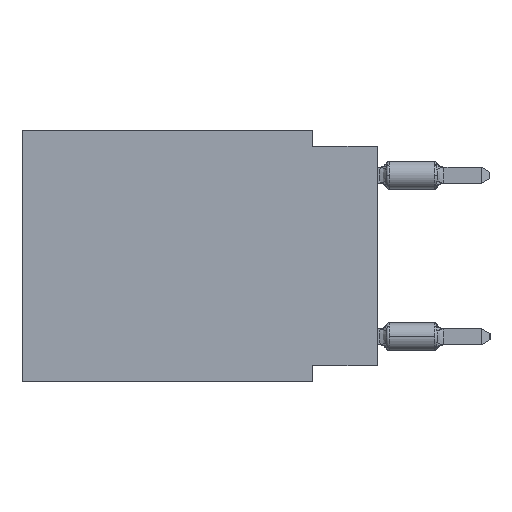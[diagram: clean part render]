
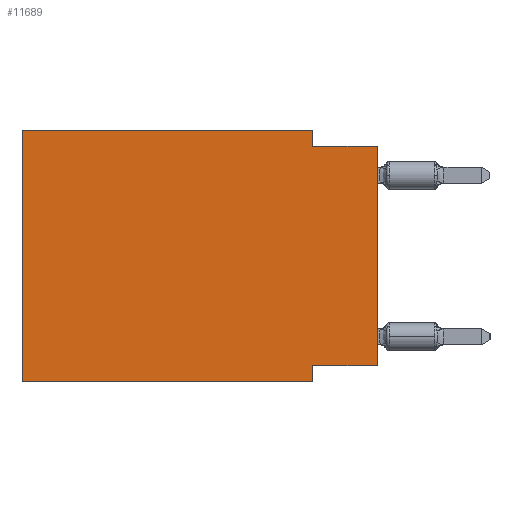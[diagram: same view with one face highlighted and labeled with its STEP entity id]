
A CAD part, left-side view. The second image highlights one B-rep face of the part: STEP entity #11689.
In plain terms, the highlighted planar face has unit normal (-1, 0, 0).
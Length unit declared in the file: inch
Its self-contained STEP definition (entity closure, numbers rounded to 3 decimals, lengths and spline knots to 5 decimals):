
#692 = LINE ( 'NONE', #32138, #29891 ) ;
#1688 = FACE_OUTER_BOUND ( 'NONE', #8664, .T. ) ;
#2341 = VERTEX_POINT ( 'NONE', #9117 ) ;
#2597 = ORIENTED_EDGE ( 'NONE', *, *, #12307, .F. ) ;
#2600 = CARTESIAN_POINT ( 'NONE',  ( 0., 0., -0.365 ) ) ;
#2831 = DIRECTION ( 'NONE',  ( 0., 0., 1. ) ) ;
#2952 = CARTESIAN_POINT ( 'NONE',  ( 0., 0., -0.025 ) ) ;
#3124 = DIRECTION ( 'NONE',  ( 0., 0., -1. ) ) ;
#4792 = VECTOR ( 'NONE', #13645, 39.37008 ) ;
#4979 = LINE ( 'NONE', #30650, #6953 ) ;
#5851 = LINE ( 'NONE', #28752, #18398 ) ;
#6953 = VECTOR ( 'NONE', #33631, 39.37008 ) ;
#7637 = VERTEX_POINT ( 'NONE', #15635 ) ;
#8664 = EDGE_LOOP ( 'NONE', ( #30148, #33648, #18701, #2597, #23044, #27809, #25547, #23635 ) ) ;
#9117 = CARTESIAN_POINT ( 'NONE',  ( 0., 0.1, -0.365 ) ) ;
#11018 = CARTESIAN_POINT ( 'NONE',  ( 0., 0.1, -0.025 ) ) ;
#11689 = ADVANCED_FACE ( 'NONE', ( #1688 ), #33144, .F. ) ;
#11784 = DIRECTION ( 'NONE',  ( 0., 1., 0. ) ) ;
#12307 = EDGE_CURVE ( 'NONE', #7637, #12621, #14099, .T. ) ;
#12621 = VERTEX_POINT ( 'NONE', #27293 ) ;
#13027 = DIRECTION ( 'NONE',  ( 0., 0., -1. ) ) ;
#13231 = CARTESIAN_POINT ( 'NONE',  ( 0., 0.1, 0. ) ) ;
#13489 = EDGE_CURVE ( 'NONE', #12621, #30700, #15653, .T. ) ;
#13645 = DIRECTION ( 'NONE',  ( 0., 0., 1. ) ) ;
#14099 = LINE ( 'NONE', #16498, #24978 ) ;
#15511 = EDGE_CURVE ( 'NONE', #30051, #30008, #692, .T. ) ;
#15635 = CARTESIAN_POINT ( 'NONE',  ( 0., 0.55, 0. ) ) ;
#15653 = LINE ( 'NONE', #13231, #29211 ) ;
#16498 = CARTESIAN_POINT ( 'NONE',  ( 0., 0.55, 0. ) ) ;
#16552 = VERTEX_POINT ( 'NONE', #2952 ) ;
#17237 = LINE ( 'NONE', #33818, #33071 ) ;
#17787 = DIRECTION ( 'NONE',  ( 0., -1., 0. ) ) ;
#18115 = CARTESIAN_POINT ( 'NONE',  ( 0., 0.55, 0. ) ) ;
#18398 = VECTOR ( 'NONE', #11784, 39.37008 ) ;
#18514 = EDGE_CURVE ( 'NONE', #30700, #16552, #4979, .T. ) ;
#18701 = ORIENTED_EDGE ( 'NONE', *, *, #13489, .F. ) ;
#19237 = CARTESIAN_POINT ( 'NONE',  ( 0., 0.55, 0. ) ) ;
#19655 = EDGE_CURVE ( 'NONE', #2341, #30008, #17237, .T. ) ;
#21150 = CARTESIAN_POINT ( 'NONE',  ( 0., 0.55, -0.39 ) ) ;
#21834 = LINE ( 'NONE', #19237, #4792 ) ;
#23044 = ORIENTED_EDGE ( 'NONE', *, *, #24681, .F. ) ;
#23635 = ORIENTED_EDGE ( 'NONE', *, *, #26785, .F. ) ;
#24681 = EDGE_CURVE ( 'NONE', #30051, #7637, #21834, .T. ) ;
#24905 = DIRECTION ( 'NONE',  ( 0., -1., 0. ) ) ;
#24948 = AXIS2_PLACEMENT_3D ( 'NONE', #18115, #29490, #13027 ) ;
#24978 = VECTOR ( 'NONE', #24905, 39.37008 ) ;
#25283 = EDGE_CURVE ( 'NONE', #25655, #16552, #28706, .T. ) ;
#25547 = ORIENTED_EDGE ( 'NONE', *, *, #19655, .F. ) ;
#25655 = VERTEX_POINT ( 'NONE', #2600 ) ;
#26785 = EDGE_CURVE ( 'NONE', #25655, #2341, #5851, .T. ) ;
#27293 = CARTESIAN_POINT ( 'NONE',  ( 0., 0.1, 0. ) ) ;
#27809 = ORIENTED_EDGE ( 'NONE', *, *, #15511, .T. ) ;
#27863 = VECTOR ( 'NONE', #2831, 39.37008 ) ;
#28332 = CARTESIAN_POINT ( 'NONE',  ( 0., 0., 0. ) ) ;
#28706 = LINE ( 'NONE', #28332, #27863 ) ;
#28752 = CARTESIAN_POINT ( 'NONE',  ( 0., 0., -0.365 ) ) ;
#29211 = VECTOR ( 'NONE', #33704, 39.37008 ) ;
#29490 = DIRECTION ( 'NONE',  ( 1., 0., 0. ) ) ;
#29891 = VECTOR ( 'NONE', #17787, 39.37008 ) ;
#30008 = VERTEX_POINT ( 'NONE', #35500 ) ;
#30051 = VERTEX_POINT ( 'NONE', #21150 ) ;
#30148 = ORIENTED_EDGE ( 'NONE', *, *, #25283, .T. ) ;
#30650 = CARTESIAN_POINT ( 'NONE',  ( 0., 0., -0.025 ) ) ;
#30700 = VERTEX_POINT ( 'NONE', #11018 ) ;
#32138 = CARTESIAN_POINT ( 'NONE',  ( 0., 0.55, -0.39 ) ) ;
#33071 = VECTOR ( 'NONE', #3124, 39.37008 ) ;
#33144 = PLANE ( 'NONE',  #24948 ) ;
#33631 = DIRECTION ( 'NONE',  ( 0., -1., 0. ) ) ;
#33648 = ORIENTED_EDGE ( 'NONE', *, *, #18514, .F. ) ;
#33704 = DIRECTION ( 'NONE',  ( 0., 0., -1. ) ) ;
#33818 = CARTESIAN_POINT ( 'NONE',  ( 0., 0.1, -0.39 ) ) ;
#35500 = CARTESIAN_POINT ( 'NONE',  ( 0., 0.1, -0.39 ) ) ;
